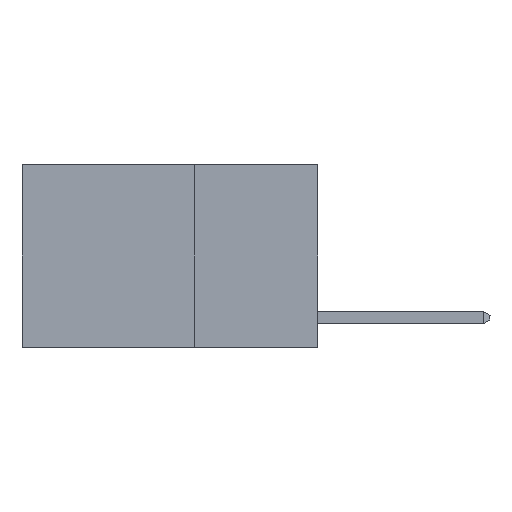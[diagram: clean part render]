
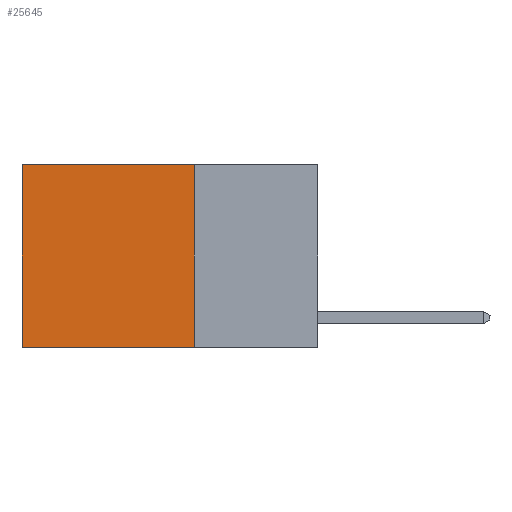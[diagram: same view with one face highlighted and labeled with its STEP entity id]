
A CAD part, left-side view. The second image highlights one B-rep face of the part: STEP entity #25645.
In plain terms, the highlighted planar face has unit normal (-1, 0, 0).
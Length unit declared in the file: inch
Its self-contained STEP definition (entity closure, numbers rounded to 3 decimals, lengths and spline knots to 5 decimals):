
#209 = VERTEX_POINT ( 'NONE', #7394 ) ;
#424 = DIRECTION ( 'NONE',  ( 0., 1., 0. ) ) ;
#934 = EDGE_CURVE ( 'NONE', #209, #24012, #26524, .T. ) ;
#1385 = ORIENTED_EDGE ( 'NONE', *, *, #934, .T. ) ;
#1931 = CARTESIAN_POINT ( 'NONE',  ( 0.2625, 0.6, -0.37 ) ) ;
#2805 = VERTEX_POINT ( 'NONE', #16053 ) ;
#6670 = CARTESIAN_POINT ( 'NONE',  ( 0.2625, 0.25, 0. ) ) ;
#6740 = CARTESIAN_POINT ( 'NONE',  ( 0.2625, 0.25, -0.37 ) ) ;
#7394 = CARTESIAN_POINT ( 'NONE',  ( 0.2625, 0.6, 0. ) ) ;
#8150 = VECTOR ( 'NONE', #424, 39.37008 ) ;
#8501 = PLANE ( 'NONE',  #14198 ) ;
#8648 = DIRECTION ( 'NONE',  ( 0., 0., -1. ) ) ;
#10280 = EDGE_CURVE ( 'NONE', #2805, #26669, #24537, .T. ) ;
#10655 = ORIENTED_EDGE ( 'NONE', *, *, #10280, .F. ) ;
#10678 = EDGE_CURVE ( 'NONE', #2805, #209, #24355, .T. ) ;
#11281 = VECTOR ( 'NONE', #19658, 39.37008 ) ;
#13216 = CARTESIAN_POINT ( 'NONE',  ( 0.2625, 0.25, 0. ) ) ;
#13463 = LINE ( 'NONE', #6740, #8150 ) ;
#14198 = AXIS2_PLACEMENT_3D ( 'NONE', #17301, #26511, #8648 ) ;
#14374 = FACE_OUTER_BOUND ( 'NONE', #19403, .T. ) ;
#14715 = VECTOR ( 'NONE', #26839, 39.37008 ) ;
#16053 = CARTESIAN_POINT ( 'NONE',  ( 0.2625, 0.25, 0. ) ) ;
#17301 = CARTESIAN_POINT ( 'NONE',  ( 0.2625, 0.25, 0. ) ) ;
#17965 = VECTOR ( 'NONE', #20157, 39.37008 ) ;
#19216 = ORIENTED_EDGE ( 'NONE', *, *, #10678, .T. ) ;
#19403 = EDGE_LOOP ( 'NONE', ( #1385, #23752, #10655, #19216 ) ) ;
#19658 = DIRECTION ( 'NONE',  ( 0., 0., -1. ) ) ;
#20157 = DIRECTION ( 'NONE',  ( 0., 0., -1. ) ) ;
#23752 = ORIENTED_EDGE ( 'NONE', *, *, #25866, .F. ) ;
#24012 = VERTEX_POINT ( 'NONE', #1931 ) ;
#24355 = LINE ( 'NONE', #13216, #14715 ) ;
#24537 = LINE ( 'NONE', #6670, #17965 ) ;
#24734 = CARTESIAN_POINT ( 'NONE',  ( 0.2625, 0.25, -0.37 ) ) ;
#25645 = ADVANCED_FACE ( 'NONE', ( #14374 ), #8501, .F. ) ;
#25866 = EDGE_CURVE ( 'NONE', #26669, #24012, #13463, .T. ) ;
#26511 = DIRECTION ( 'NONE',  ( 1., 0., 0. ) ) ;
#26524 = LINE ( 'NONE', #26815, #11281 ) ;
#26669 = VERTEX_POINT ( 'NONE', #24734 ) ;
#26815 = CARTESIAN_POINT ( 'NONE',  ( 0.2625, 0.6, 0. ) ) ;
#26839 = DIRECTION ( 'NONE',  ( 0., 1., 0. ) ) ;
